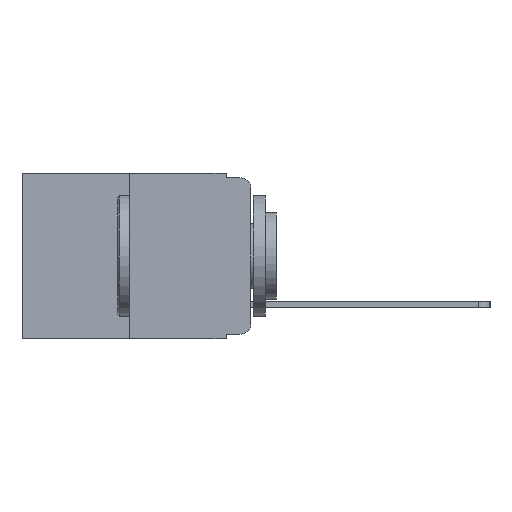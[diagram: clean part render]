
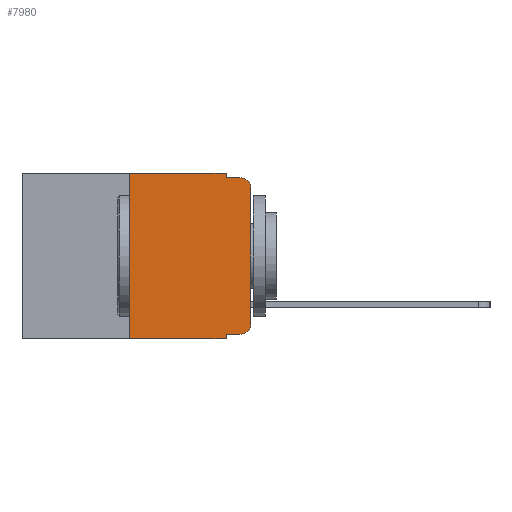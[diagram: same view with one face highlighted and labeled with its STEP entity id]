
A CAD part, left-side view. The second image highlights one B-rep face of the part: STEP entity #7980.
In plain terms, the highlighted planar face has unit normal (-1, 0, 0).
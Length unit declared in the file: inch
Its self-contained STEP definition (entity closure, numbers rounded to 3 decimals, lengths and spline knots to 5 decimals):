
#54 = LINE ( 'NONE', #6568, #14674 ) ;
#142 = DIRECTION ( 'NONE',  ( -1., 0., 0. ) ) ;
#260 = ORIENTED_EDGE ( 'NONE', *, *, #2645, .F. ) ;
#1037 = DIRECTION ( 'NONE',  ( 0., 0., -1. ) ) ;
#1265 = DIRECTION ( 'NONE',  ( 0., -1., 0. ) ) ;
#1286 = ORIENTED_EDGE ( 'NONE', *, *, #2677, .T. ) ;
#1444 = EDGE_CURVE ( 'NONE', #12956, #13489, #54, .T. ) ;
#1495 = VERTEX_POINT ( 'NONE', #7522 ) ;
#1675 = CARTESIAN_POINT ( 'NONE',  ( 0., 0.473, 0. ) ) ;
#2592 = EDGE_CURVE ( 'NONE', #1495, #14700, #18377, .T. ) ;
#2613 = EDGE_CURVE ( 'NONE', #14700, #14209, #3306, .T. ) ;
#2619 = EDGE_CURVE ( 'NONE', #9426, #14209, #14642, .T. ) ;
#2622 = EDGE_CURVE ( 'NONE', #13992, #9426, #7181, .T. ) ;
#2643 = EDGE_CURVE ( 'NONE', #12956, #18711, #10206, .T. ) ;
#2645 = EDGE_CURVE ( 'NONE', #7134, #13489, #13832, .T. ) ;
#2670 = EDGE_CURVE ( 'NONE', #7134, #9521, #17251, .T. ) ;
#2677 = EDGE_CURVE ( 'NONE', #9521, #1495, #9769, .T. ) ;
#2778 = CARTESIAN_POINT ( 'NONE',  ( 0., 0.051, -0.01 ) ) ;
#3006 = AXIS2_PLACEMENT_3D ( 'NONE', #13188, #10458, #1037 ) ;
#3306 = CIRCLE ( 'NONE', #9950, 0.02 ) ;
#3525 = DIRECTION ( 'NONE',  ( 0., -1., 0. ) ) ;
#4351 = DIRECTION ( 'NONE',  ( 0., 0., -1. ) ) ;
#4699 = EDGE_CURVE ( 'NONE', #18711, #13992, #18586, .T. ) ;
#5470 = CARTESIAN_POINT ( 'NONE',  ( 0., 0.051, 0. ) ) ;
#6207 = VECTOR ( 'NONE', #13505, 39.37008 ) ;
#6568 = CARTESIAN_POINT ( 'NONE',  ( 0., 0.473, -0.343 ) ) ;
#6601 = CARTESIAN_POINT ( 'NONE',  ( 0., 0.051, -0.333 ) ) ;
#6709 = VECTOR ( 'NONE', #13854, 39.37008 ) ;
#6977 = CARTESIAN_POINT ( 'NONE',  ( 0., 0.25, 0. ) ) ;
#7134 = VERTEX_POINT ( 'NONE', #7399 ) ;
#7181 = LINE ( 'NONE', #5470, #10621 ) ;
#7204 = CARTESIAN_POINT ( 'NONE',  ( 0., 0.02, -0.333 ) ) ;
#7399 = CARTESIAN_POINT ( 'NONE',  ( 0., 0.051, -0.333 ) ) ;
#7400 = ORIENTED_EDGE ( 'NONE', *, *, #4699, .F. ) ;
#7410 = CARTESIAN_POINT ( 'NONE',  ( 0., 0.051, -0.343 ) ) ;
#7522 = CARTESIAN_POINT ( 'NONE',  ( 0., 0., -0.313 ) ) ;
#7924 = VECTOR ( 'NONE', #1265, 39.37008 ) ;
#7980 = ADVANCED_FACE ( 'NONE', ( #13905 ), #14476, .F. ) ;
#8708 = CARTESIAN_POINT ( 'NONE',  ( 0., 0.02, -0.03 ) ) ;
#9426 = VERTEX_POINT ( 'NONE', #17847 ) ;
#9497 = CARTESIAN_POINT ( 'NONE',  ( 0., 0.25, -0.343 ) ) ;
#9521 = VERTEX_POINT ( 'NONE', #7204 ) ;
#9634 = EDGE_LOOP ( 'NONE', ( #10409, #17432, #14428, #17821, #7400, #11739, #15296, #260, #12600, #1286 ) ) ;
#9769 = CIRCLE ( 'NONE', #10856, 0.02 ) ;
#9950 = AXIS2_PLACEMENT_3D ( 'NONE', #8708, #142, #16425 ) ;
#10206 = LINE ( 'NONE', #16090, #6207 ) ;
#10409 = ORIENTED_EDGE ( 'NONE', *, *, #2592, .T. ) ;
#10458 = DIRECTION ( 'NONE',  ( 1., 0., 0. ) ) ;
#10503 = DIRECTION ( 'NONE',  ( 0., 0., -1. ) ) ;
#10621 = VECTOR ( 'NONE', #10503, 39.37008 ) ;
#10856 = AXIS2_PLACEMENT_3D ( 'NONE', #12902, #15810, #4351 ) ;
#10976 = CARTESIAN_POINT ( 'NONE',  ( 0., 0.051, 0. ) ) ;
#11076 = VECTOR ( 'NONE', #11180, 39.37008 ) ;
#11180 = DIRECTION ( 'NONE',  ( 0., 0., 1. ) ) ;
#11198 = DIRECTION ( 'NONE',  ( 0., -1., 0. ) ) ;
#11714 = DIRECTION ( 'NONE',  ( 0., -1., 0. ) ) ;
#11739 = ORIENTED_EDGE ( 'NONE', *, *, #2643, .F. ) ;
#12198 = CARTESIAN_POINT ( 'NONE',  ( 0., 0., 0. ) ) ;
#12600 = ORIENTED_EDGE ( 'NONE', *, *, #2670, .T. ) ;
#12883 = CARTESIAN_POINT ( 'NONE',  ( 0., 0., -0.03 ) ) ;
#12902 = CARTESIAN_POINT ( 'NONE',  ( 0., 0.02, -0.313 ) ) ;
#12956 = VERTEX_POINT ( 'NONE', #9497 ) ;
#13188 = CARTESIAN_POINT ( 'NONE',  ( 0., 0.473, 0. ) ) ;
#13278 = CARTESIAN_POINT ( 'NONE',  ( 0., 0.051, 0. ) ) ;
#13489 = VERTEX_POINT ( 'NONE', #7410 ) ;
#13505 = DIRECTION ( 'NONE',  ( 0., 0., 1. ) ) ;
#13832 = LINE ( 'NONE', #13278, #6709 ) ;
#13854 = DIRECTION ( 'NONE',  ( 0., 0., -1. ) ) ;
#13905 = FACE_OUTER_BOUND ( 'NONE', #9634, .T. ) ;
#13992 = VERTEX_POINT ( 'NONE', #10976 ) ;
#14209 = VERTEX_POINT ( 'NONE', #16944 ) ;
#14244 = VECTOR ( 'NONE', #3525, 39.37008 ) ;
#14428 = ORIENTED_EDGE ( 'NONE', *, *, #2619, .F. ) ;
#14476 = PLANE ( 'NONE',  #3006 ) ;
#14642 = LINE ( 'NONE', #2778, #17626 ) ;
#14674 = VECTOR ( 'NONE', #11714, 39.37008 ) ;
#14700 = VERTEX_POINT ( 'NONE', #12883 ) ;
#15296 = ORIENTED_EDGE ( 'NONE', *, *, #1444, .T. ) ;
#15810 = DIRECTION ( 'NONE',  ( -1., 0., 0. ) ) ;
#16090 = CARTESIAN_POINT ( 'NONE',  ( 0., 0.25, 0. ) ) ;
#16425 = DIRECTION ( 'NONE',  ( 0., 0., -1. ) ) ;
#16944 = CARTESIAN_POINT ( 'NONE',  ( 0., 0.02, -0.01 ) ) ;
#17251 = LINE ( 'NONE', #6601, #14244 ) ;
#17432 = ORIENTED_EDGE ( 'NONE', *, *, #2613, .T. ) ;
#17626 = VECTOR ( 'NONE', #11198, 39.37008 ) ;
#17821 = ORIENTED_EDGE ( 'NONE', *, *, #2622, .F. ) ;
#17847 = CARTESIAN_POINT ( 'NONE',  ( 0., 0.051, -0.01 ) ) ;
#18377 = LINE ( 'NONE', #12198, #11076 ) ;
#18586 = LINE ( 'NONE', #1675, #7924 ) ;
#18711 = VERTEX_POINT ( 'NONE', #6977 ) ;
